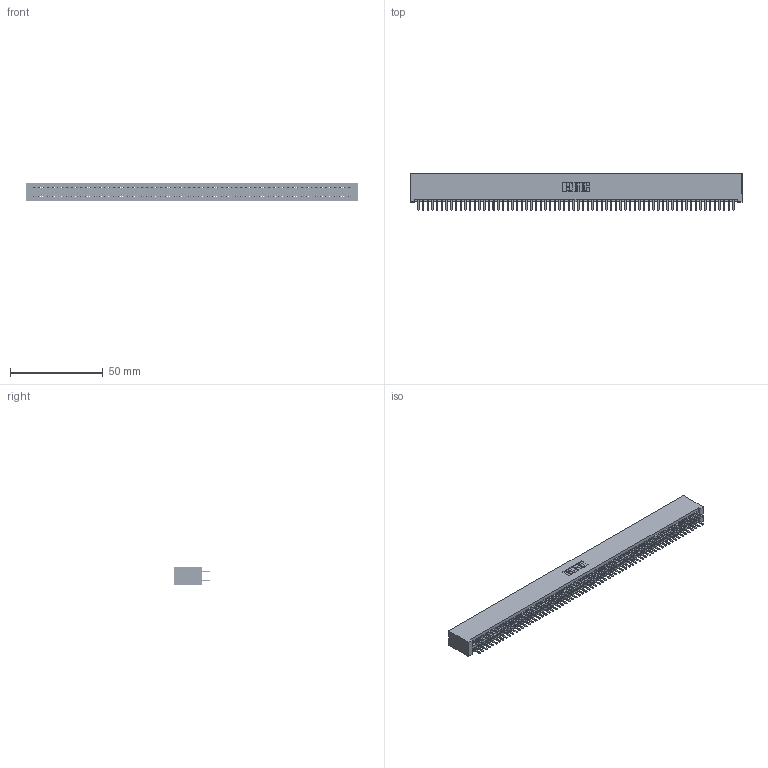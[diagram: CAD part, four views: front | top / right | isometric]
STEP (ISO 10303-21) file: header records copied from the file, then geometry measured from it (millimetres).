
FILE_DESCRIPTION (( 'STEP AP203' ), '1' );
FILE_NAME ('395-136-520-201.STEP', '2018-12-05T06:23:50', ( '' ), ( '' ), 'SwSTEP 2.0', 'SolidWorks 2016', '' );
FILE_SCHEMA (( 'CONFIG_CONTROL_DESIGN' ));
Length unit declared in the file: inch
Products named in the file (3): 345-292-001_345-293-120; 395-136-520-201; 345 Part_No Mounting Lugs
Assembly tree (137 placements, depth 2):
  395-136-520-201
    345 Part_No Mounting Lugs
    345-292-001_345-293-120  x136
Bounding box: 179.32 x 19.68 x 9.4 mm (x, y, z)
Volume: 18217.2 mm3; surface area: 27607.7 mm2
Topology: 137 solids, 137 shells, 7462 faces, 21669 edges, 14082 vertices
Faces by surface type: plane 4836, cylinder 2626
Entity records: 49691 total; most frequent: CARTESIAN_POINT 8316, ORIENTED_EDGE 8238, DIRECTION 7283, EDGE_CURVE 4119, VECTOR 3719, LINE 3719, VERTEX_POINT 2742, AXIS2_PLACEMENT_3D 1782
